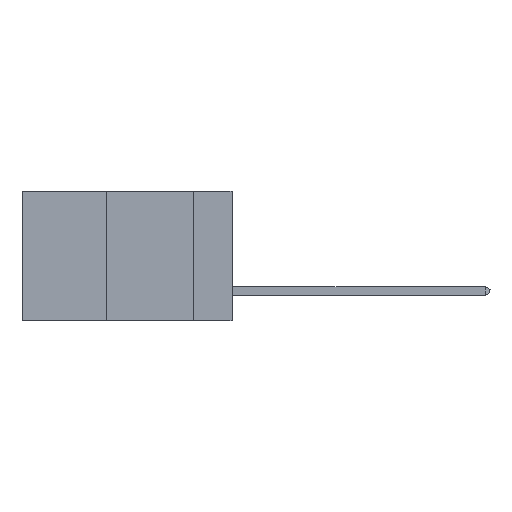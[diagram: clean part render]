
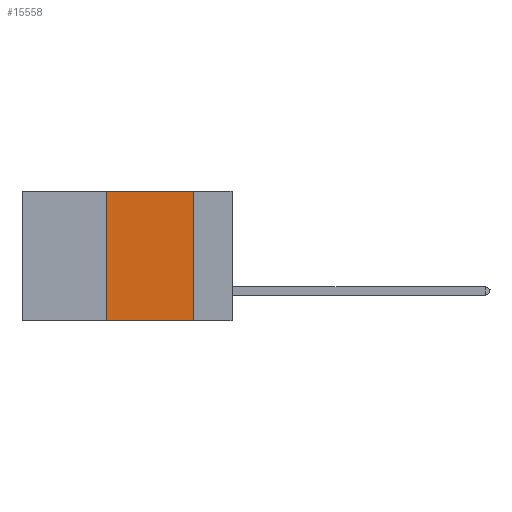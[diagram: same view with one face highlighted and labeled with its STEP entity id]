
A CAD part, left-side view. The second image highlights one B-rep face of the part: STEP entity #15558.
In plain terms, the highlighted planar face has unit normal (-1, 0, 0).
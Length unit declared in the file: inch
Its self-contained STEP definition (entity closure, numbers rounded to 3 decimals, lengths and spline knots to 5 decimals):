
#160 = EDGE_CURVE ( 'NONE', #15401, #8781, #10901, .T. ) ;
#432 = DIRECTION ( 'NONE',  ( 0., -1., 0. ) ) ;
#1720 = VECTOR ( 'NONE', #8478, 39.37008 ) ;
#2309 = ORIENTED_EDGE ( 'NONE', *, *, #15620, .F. ) ;
#2959 = CARTESIAN_POINT ( 'NONE',  ( 0., 0.6, 0. ) ) ;
#3909 = EDGE_CURVE ( 'NONE', #16574, #8270, #16532, .T. ) ;
#4538 = VECTOR ( 'NONE', #4560, 39.37008 ) ;
#4560 = DIRECTION ( 'NONE',  ( 0., 0., -1. ) ) ;
#5197 = CARTESIAN_POINT ( 'NONE',  ( 0., 0.36, -0.37 ) ) ;
#6204 = EDGE_LOOP ( 'NONE', ( #16967, #2309, #17993, #8675 ) ) ;
#7415 = CARTESIAN_POINT ( 'NONE',  ( 0., 0.11, -0.37 ) ) ;
#7850 = DIRECTION ( 'NONE',  ( 0., -1., 0. ) ) ;
#8270 = VERTEX_POINT ( 'NONE', #7415 ) ;
#8478 = DIRECTION ( 'NONE',  ( 0., 0., 1. ) ) ;
#8675 = ORIENTED_EDGE ( 'NONE', *, *, #14374, .T. ) ;
#8781 = VERTEX_POINT ( 'NONE', #13291 ) ;
#9896 = VECTOR ( 'NONE', #432, 39.37008 ) ;
#10191 = VECTOR ( 'NONE', #7850, 39.37008 ) ;
#10901 = LINE ( 'NONE', #16144, #1720 ) ;
#11725 = LINE ( 'NONE', #18395, #9896 ) ;
#11737 = CARTESIAN_POINT ( 'NONE',  ( 0., 0.11, 0. ) ) ;
#12710 = PLANE ( 'NONE',  #16711 ) ;
#13291 = CARTESIAN_POINT ( 'NONE',  ( 0., 0.36, 0. ) ) ;
#14335 = DIRECTION ( 'NONE',  ( 0., 0., -1. ) ) ;
#14374 = EDGE_CURVE ( 'NONE', #15401, #8270, #11725, .T. ) ;
#15031 = CARTESIAN_POINT ( 'NONE',  ( 0., 0.11, 0. ) ) ;
#15401 = VERTEX_POINT ( 'NONE', #5197 ) ;
#15558 = ADVANCED_FACE ( 'NONE', ( #16037 ), #12710, .F. ) ;
#15620 = EDGE_CURVE ( 'NONE', #8781, #16574, #20084, .T. ) ;
#15825 = DIRECTION ( 'NONE',  ( 1., 0., 0. ) ) ;
#16037 = FACE_OUTER_BOUND ( 'NONE', #6204, .T. ) ;
#16144 = CARTESIAN_POINT ( 'NONE',  ( 0., 0.36, 0. ) ) ;
#16532 = LINE ( 'NONE', #11737, #4538 ) ;
#16574 = VERTEX_POINT ( 'NONE', #15031 ) ;
#16711 = AXIS2_PLACEMENT_3D ( 'NONE', #2959, #15825, #14335 ) ;
#16967 = ORIENTED_EDGE ( 'NONE', *, *, #3909, .F. ) ;
#17609 = CARTESIAN_POINT ( 'NONE',  ( 0., 0.6, 0. ) ) ;
#17993 = ORIENTED_EDGE ( 'NONE', *, *, #160, .F. ) ;
#18395 = CARTESIAN_POINT ( 'NONE',  ( 0., 0.6, -0.37 ) ) ;
#20084 = LINE ( 'NONE', #17609, #10191 ) ;
